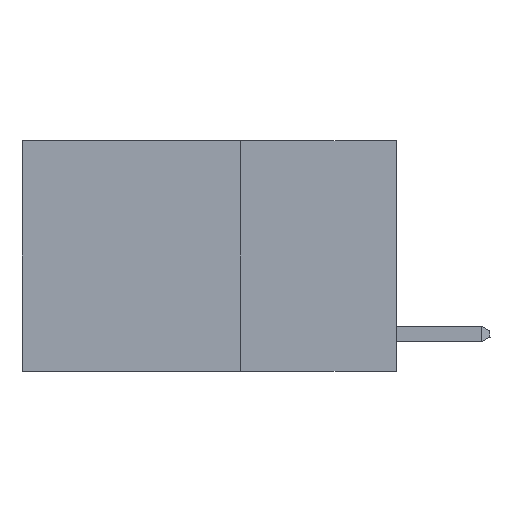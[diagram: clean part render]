
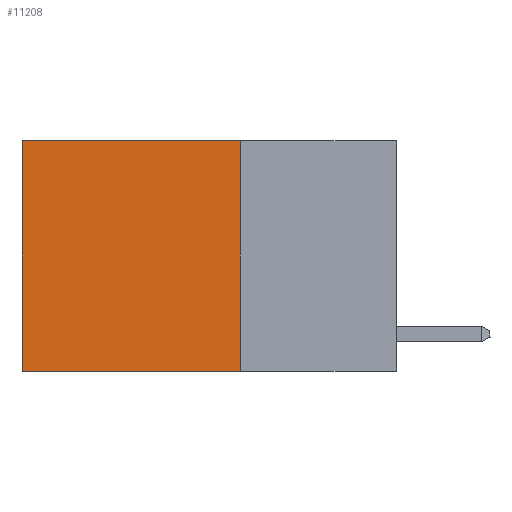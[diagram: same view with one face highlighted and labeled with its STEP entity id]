
A CAD part, left-side view. The second image highlights one B-rep face of the part: STEP entity #11208.
In plain terms, the highlighted planar face has unit normal (-1, 0, 0).
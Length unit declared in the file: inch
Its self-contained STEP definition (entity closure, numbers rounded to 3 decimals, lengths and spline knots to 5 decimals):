
#687 = VECTOR ( 'NONE', #5611, 39.37008 ) ;
#1310 = VERTEX_POINT ( 'NONE', #13130 ) ;
#1391 = FACE_OUTER_BOUND ( 'NONE', #12167, .T. ) ;
#1439 = CARTESIAN_POINT ( 'NONE',  ( 0.2625, 0.6, 0. ) ) ;
#1989 = CARTESIAN_POINT ( 'NONE',  ( 0.2625, 0.25, 0. ) ) ;
#4466 = LINE ( 'NONE', #1989, #17023 ) ;
#4797 = EDGE_CURVE ( 'NONE', #7080, #1310, #14663, .T. ) ;
#4997 = ORIENTED_EDGE ( 'NONE', *, *, #20529, .F. ) ;
#5611 = DIRECTION ( 'NONE',  ( 0., 1., 0. ) ) ;
#5931 = CARTESIAN_POINT ( 'NONE',  ( 0.2625, 0.25, 0. ) ) ;
#7080 = VERTEX_POINT ( 'NONE', #5931 ) ;
#7306 = VECTOR ( 'NONE', #10809, 39.37008 ) ;
#7422 = LINE ( 'NONE', #15153, #687 ) ;
#8557 = ORIENTED_EDGE ( 'NONE', *, *, #4797, .T. ) ;
#9151 = CARTESIAN_POINT ( 'NONE',  ( 0.2625, 0.25, -0.37 ) ) ;
#9334 = DIRECTION ( 'NONE',  ( 0., 0., -1. ) ) ;
#10809 = DIRECTION ( 'NONE',  ( 0., 1., 0. ) ) ;
#11020 = VECTOR ( 'NONE', #9334, 39.37008 ) ;
#11208 = ADVANCED_FACE ( 'NONE', ( #1391 ), #23476, .F. ) ;
#11337 = CARTESIAN_POINT ( 'NONE',  ( 0.2625, 0.25, 0. ) ) ;
#12167 = EDGE_LOOP ( 'NONE', ( #19857, #4997, #23366, #8557 ) ) ;
#13062 = EDGE_CURVE ( 'NONE', #7080, #20038, #4466, .T. ) ;
#13130 = CARTESIAN_POINT ( 'NONE',  ( 0.2625, 0.6, 0. ) ) ;
#13998 = DIRECTION ( 'NONE',  ( 0., 0., -1. ) ) ;
#14663 = LINE ( 'NONE', #24884, #7306 ) ;
#15153 = CARTESIAN_POINT ( 'NONE',  ( 0.2625, 0.25, -0.37 ) ) ;
#17023 = VECTOR ( 'NONE', #13998, 39.37008 ) ;
#19033 = AXIS2_PLACEMENT_3D ( 'NONE', #11337, #19323, #25029 ) ;
#19323 = DIRECTION ( 'NONE',  ( 1., 0., 0. ) ) ;
#19857 = ORIENTED_EDGE ( 'NONE', *, *, #21054, .T. ) ;
#20038 = VERTEX_POINT ( 'NONE', #9151 ) ;
#20529 = EDGE_CURVE ( 'NONE', #20038, #23075, #7422, .T. ) ;
#21054 = EDGE_CURVE ( 'NONE', #1310, #23075, #23755, .T. ) ;
#23075 = VERTEX_POINT ( 'NONE', #24722 ) ;
#23366 = ORIENTED_EDGE ( 'NONE', *, *, #13062, .F. ) ;
#23476 = PLANE ( 'NONE',  #19033 ) ;
#23755 = LINE ( 'NONE', #1439, #11020 ) ;
#24722 = CARTESIAN_POINT ( 'NONE',  ( 0.2625, 0.6, -0.37 ) ) ;
#24884 = CARTESIAN_POINT ( 'NONE',  ( 0.2625, 0.25, 0. ) ) ;
#25029 = DIRECTION ( 'NONE',  ( 0., 0., -1. ) ) ;
